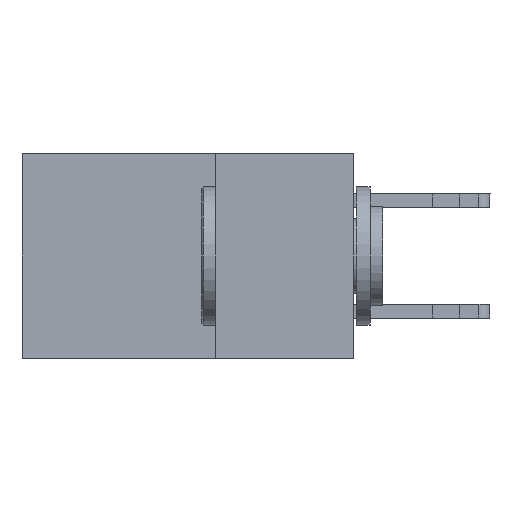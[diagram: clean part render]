
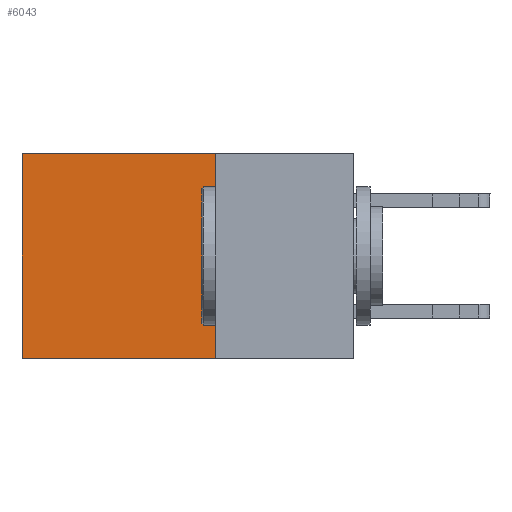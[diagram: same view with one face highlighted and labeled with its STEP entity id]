
A CAD part, left-side view. The second image highlights one B-rep face of the part: STEP entity #6043.
In plain terms, the highlighted planar face has unit normal (-1, 0, 0).
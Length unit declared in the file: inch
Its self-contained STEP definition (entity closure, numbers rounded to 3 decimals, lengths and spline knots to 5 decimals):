
#1064 = VERTEX_POINT ( 'NONE', #6553 ) ;
#1899 = VERTEX_POINT ( 'NONE', #29283 ) ;
#2069 = LINE ( 'NONE', #18455, #2892 ) ;
#2892 = VECTOR ( 'NONE', #21014, 39.37008 ) ;
#3096 = EDGE_CURVE ( 'NONE', #30346, #1899, #2069, .T. ) ;
#3566 = EDGE_CURVE ( 'NONE', #1064, #1899, #14402, .T. ) ;
#5046 = DIRECTION ( 'NONE',  ( 0., 0., -1. ) ) ;
#5481 = CARTESIAN_POINT ( 'NONE',  ( 0.2875, 0.25, -0.37 ) ) ;
#6043 = ADVANCED_FACE ( 'NONE', ( #14819 ), #17423, .F. ) ;
#6553 = CARTESIAN_POINT ( 'NONE',  ( 0.2875, 0.25, -0.37 ) ) ;
#7100 = AXIS2_PLACEMENT_3D ( 'NONE', #22957, #7121, #5046 ) ;
#7121 = DIRECTION ( 'NONE',  ( 1., 0., 0. ) ) ;
#7370 = ORIENTED_EDGE ( 'NONE', *, *, #22224, .T. ) ;
#11753 = CARTESIAN_POINT ( 'NONE',  ( 0.2875, 0.25, 0. ) ) ;
#13333 = ORIENTED_EDGE ( 'NONE', *, *, #3566, .F. ) ;
#14402 = LINE ( 'NONE', #5481, #18953 ) ;
#14819 = FACE_OUTER_BOUND ( 'NONE', #29638, .T. ) ;
#15488 = EDGE_CURVE ( 'NONE', #28780, #1064, #29258, .T. ) ;
#17423 = PLANE ( 'NONE',  #7100 ) ;
#18455 = CARTESIAN_POINT ( 'NONE',  ( 0.2875, 0.6, 0. ) ) ;
#18953 = VECTOR ( 'NONE', #23977, 39.37008 ) ;
#19790 = DIRECTION ( 'NONE',  ( 0., 1., 0. ) ) ;
#21014 = DIRECTION ( 'NONE',  ( 0., 0., -1. ) ) ;
#22224 = EDGE_CURVE ( 'NONE', #28780, #30346, #26877, .T. ) ;
#22799 = DIRECTION ( 'NONE',  ( 0., 0., -1. ) ) ;
#22957 = CARTESIAN_POINT ( 'NONE',  ( 0.2875, 0.25, 0. ) ) ;
#23153 = CARTESIAN_POINT ( 'NONE',  ( 0.2875, 0.25, 0. ) ) ;
#23977 = DIRECTION ( 'NONE',  ( 0., 1., 0. ) ) ;
#25641 = VECTOR ( 'NONE', #19790, 39.37008 ) ;
#26088 = ORIENTED_EDGE ( 'NONE', *, *, #3096, .T. ) ;
#26877 = LINE ( 'NONE', #11753, #25641 ) ;
#28415 = VECTOR ( 'NONE', #22799, 39.37008 ) ;
#28780 = VERTEX_POINT ( 'NONE', #29061 ) ;
#29061 = CARTESIAN_POINT ( 'NONE',  ( 0.2875, 0.25, 0. ) ) ;
#29258 = LINE ( 'NONE', #23153, #28415 ) ;
#29283 = CARTESIAN_POINT ( 'NONE',  ( 0.2875, 0.6, -0.37 ) ) ;
#29638 = EDGE_LOOP ( 'NONE', ( #26088, #13333, #30499, #7370 ) ) ;
#30346 = VERTEX_POINT ( 'NONE', #33114 ) ;
#30499 = ORIENTED_EDGE ( 'NONE', *, *, #15488, .F. ) ;
#33114 = CARTESIAN_POINT ( 'NONE',  ( 0.2875, 0.6, 0. ) ) ;
